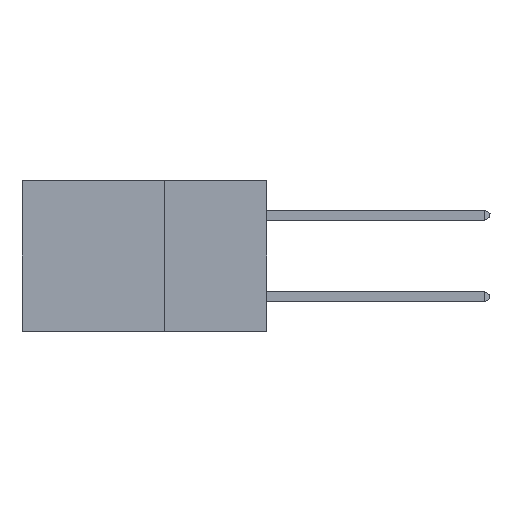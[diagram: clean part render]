
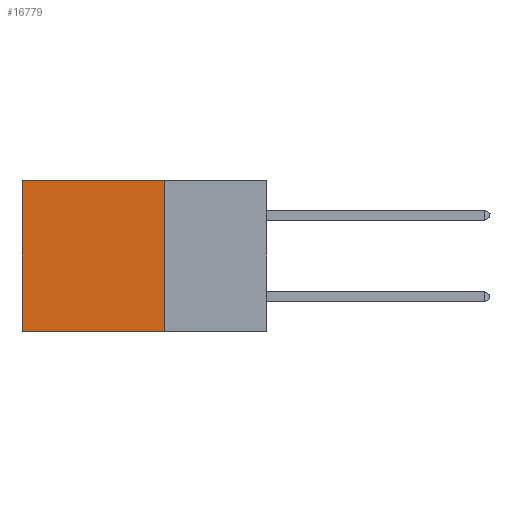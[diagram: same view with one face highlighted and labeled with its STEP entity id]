
A CAD part, left-side view. The second image highlights one B-rep face of the part: STEP entity #16779.
In plain terms, the highlighted planar face has unit normal (-1, 0, 0).
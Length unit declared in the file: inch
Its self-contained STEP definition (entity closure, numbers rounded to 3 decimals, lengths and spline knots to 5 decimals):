
#302 = VECTOR ( 'NONE', #6375, 39.37008 ) ;
#322 = CARTESIAN_POINT ( 'NONE',  ( 0.2875, 0.25, 0. ) ) ;
#1150 = VECTOR ( 'NONE', #11214, 39.37008 ) ;
#1252 = CARTESIAN_POINT ( 'NONE',  ( 0.2875, 0.6, -0.37 ) ) ;
#1593 = VECTOR ( 'NONE', #3018, 39.37008 ) ;
#3018 = DIRECTION ( 'NONE',  ( 0., 0., -1. ) ) ;
#3709 = LINE ( 'NONE', #8568, #302 ) ;
#3803 = AXIS2_PLACEMENT_3D ( 'NONE', #8044, #5693, #10737 ) ;
#3951 = ORIENTED_EDGE ( 'NONE', *, *, #27509, .F. ) ;
#5693 = DIRECTION ( 'NONE',  ( 1., 0., 0. ) ) ;
#6375 = DIRECTION ( 'NONE',  ( 0., 1., 0. ) ) ;
#7997 = VERTEX_POINT ( 'NONE', #1252 ) ;
#8044 = CARTESIAN_POINT ( 'NONE',  ( 0.2875, 0.25, 0. ) ) ;
#8399 = ORIENTED_EDGE ( 'NONE', *, *, #25923, .F. ) ;
#8568 = CARTESIAN_POINT ( 'NONE',  ( 0.2875, 0.25, 0. ) ) ;
#8759 = EDGE_LOOP ( 'NONE', ( #25290, #8399, #3951, #12642 ) ) ;
#9963 = LINE ( 'NONE', #24493, #11293 ) ;
#10020 = PLANE ( 'NONE',  #3803 ) ;
#10623 = LINE ( 'NONE', #11183, #1593 ) ;
#10737 = DIRECTION ( 'NONE',  ( 0., 0., -1. ) ) ;
#11183 = CARTESIAN_POINT ( 'NONE',  ( 0.2875, 0.6, 0. ) ) ;
#11214 = DIRECTION ( 'NONE',  ( 0., 0., -1. ) ) ;
#11293 = VECTOR ( 'NONE', #11631, 39.37008 ) ;
#11631 = DIRECTION ( 'NONE',  ( 0., 1., 0. ) ) ;
#12642 = ORIENTED_EDGE ( 'NONE', *, *, #19949, .T. ) ;
#13881 = CARTESIAN_POINT ( 'NONE',  ( 0.2875, 0.6, 0. ) ) ;
#14061 = CARTESIAN_POINT ( 'NONE',  ( 0.2875, 0.25, -0.37 ) ) ;
#14594 = LINE ( 'NONE', #322, #1150 ) ;
#16779 = ADVANCED_FACE ( 'NONE', ( #18970 ), #10020, .F. ) ;
#18956 = VERTEX_POINT ( 'NONE', #13881 ) ;
#18970 = FACE_OUTER_BOUND ( 'NONE', #8759, .T. ) ;
#19949 = EDGE_CURVE ( 'NONE', #25055, #18956, #3709, .T. ) ;
#23568 = CARTESIAN_POINT ( 'NONE',  ( 0.2875, 0.25, 0. ) ) ;
#23886 = VERTEX_POINT ( 'NONE', #14061 ) ;
#24493 = CARTESIAN_POINT ( 'NONE',  ( 0.2875, 0.25, -0.37 ) ) ;
#25055 = VERTEX_POINT ( 'NONE', #23568 ) ;
#25290 = ORIENTED_EDGE ( 'NONE', *, *, #26237, .T. ) ;
#25923 = EDGE_CURVE ( 'NONE', #23886, #7997, #9963, .T. ) ;
#26237 = EDGE_CURVE ( 'NONE', #18956, #7997, #10623, .T. ) ;
#27509 = EDGE_CURVE ( 'NONE', #25055, #23886, #14594, .T. ) ;
